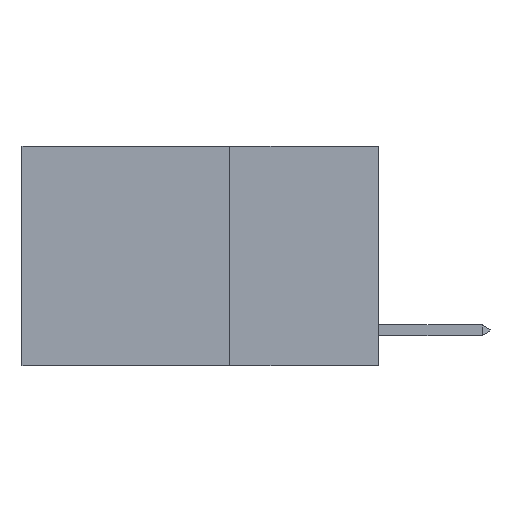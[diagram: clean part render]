
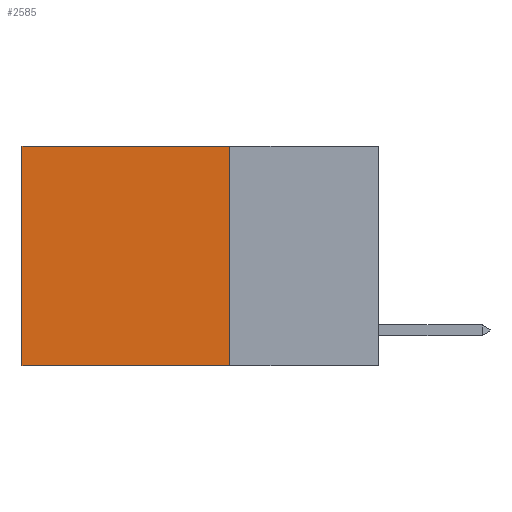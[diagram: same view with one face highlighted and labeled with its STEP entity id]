
A CAD part, left-side view. The second image highlights one B-rep face of the part: STEP entity #2585.
In plain terms, the highlighted planar face has unit normal (-1, 0, 0).
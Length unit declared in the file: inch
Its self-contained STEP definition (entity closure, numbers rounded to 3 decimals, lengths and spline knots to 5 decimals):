
#176 = CARTESIAN_POINT ( 'NONE',  ( 0.2625, 0.25, 0. ) ) ;
#2010 = VERTEX_POINT ( 'NONE', #5437 ) ;
#2299 = DIRECTION ( 'NONE',  ( 0., 0., -1. ) ) ;
#2455 = LINE ( 'NONE', #21745, #6110 ) ;
#2585 = ADVANCED_FACE ( 'NONE', ( #17648 ), #8572, .F. ) ;
#3283 = CARTESIAN_POINT ( 'NONE',  ( 0.2625, 0.25, 0. ) ) ;
#3667 = VECTOR ( 'NONE', #8762, 39.37008 ) ;
#3768 = ORIENTED_EDGE ( 'NONE', *, *, #6476, .T. ) ;
#4625 = VERTEX_POINT ( 'NONE', #13177 ) ;
#5108 = DIRECTION ( 'NONE',  ( 0., 0., -1. ) ) ;
#5437 = CARTESIAN_POINT ( 'NONE',  ( 0.2625, 0.6, -0.37 ) ) ;
#6110 = VECTOR ( 'NONE', #2299, 39.37008 ) ;
#6476 = EDGE_CURVE ( 'NONE', #4625, #2010, #2455, .T. ) ;
#7090 = VERTEX_POINT ( 'NONE', #9382 ) ;
#7576 = AXIS2_PLACEMENT_3D ( 'NONE', #3283, #15729, #5108 ) ;
#7671 = DIRECTION ( 'NONE',  ( 0., 0., -1. ) ) ;
#8120 = LINE ( 'NONE', #12951, #22755 ) ;
#8572 = PLANE ( 'NONE',  #7576 ) ;
#8762 = DIRECTION ( 'NONE',  ( 0., 1., 0. ) ) ;
#9338 = LINE ( 'NONE', #176, #18177 ) ;
#9382 = CARTESIAN_POINT ( 'NONE',  ( 0.2625, 0.25, 0. ) ) ;
#12430 = ORIENTED_EDGE ( 'NONE', *, *, #15497, .F. ) ;
#12693 = DIRECTION ( 'NONE',  ( 0., 1., 0. ) ) ;
#12951 = CARTESIAN_POINT ( 'NONE',  ( 0.2625, 0.25, 0. ) ) ;
#13131 = LINE ( 'NONE', #22801, #3667 ) ;
#13174 = VERTEX_POINT ( 'NONE', #21664 ) ;
#13177 = CARTESIAN_POINT ( 'NONE',  ( 0.2625, 0.6, 0. ) ) ;
#13319 = EDGE_LOOP ( 'NONE', ( #3768, #12430, #19778, #18501 ) ) ;
#15497 = EDGE_CURVE ( 'NONE', #13174, #2010, #13131, .T. ) ;
#15729 = DIRECTION ( 'NONE',  ( 1., 0., 0. ) ) ;
#15730 = EDGE_CURVE ( 'NONE', #7090, #13174, #8120, .T. ) ;
#17648 = FACE_OUTER_BOUND ( 'NONE', #13319, .T. ) ;
#18177 = VECTOR ( 'NONE', #12693, 39.37008 ) ;
#18501 = ORIENTED_EDGE ( 'NONE', *, *, #19167, .T. ) ;
#19167 = EDGE_CURVE ( 'NONE', #7090, #4625, #9338, .T. ) ;
#19778 = ORIENTED_EDGE ( 'NONE', *, *, #15730, .F. ) ;
#21664 = CARTESIAN_POINT ( 'NONE',  ( 0.2625, 0.25, -0.37 ) ) ;
#21745 = CARTESIAN_POINT ( 'NONE',  ( 0.2625, 0.6, 0. ) ) ;
#22755 = VECTOR ( 'NONE', #7671, 39.37008 ) ;
#22801 = CARTESIAN_POINT ( 'NONE',  ( 0.2625, 0.25, -0.37 ) ) ;
